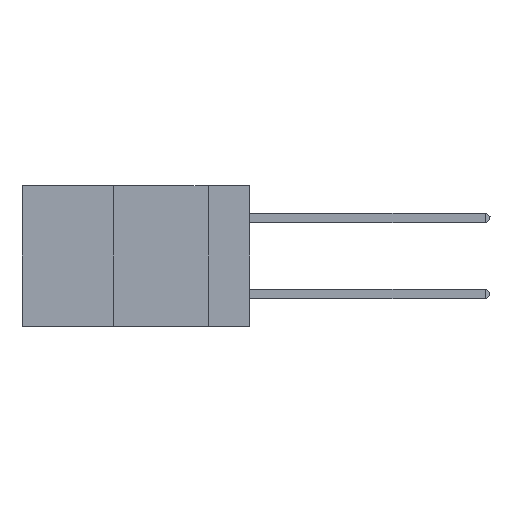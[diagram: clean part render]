
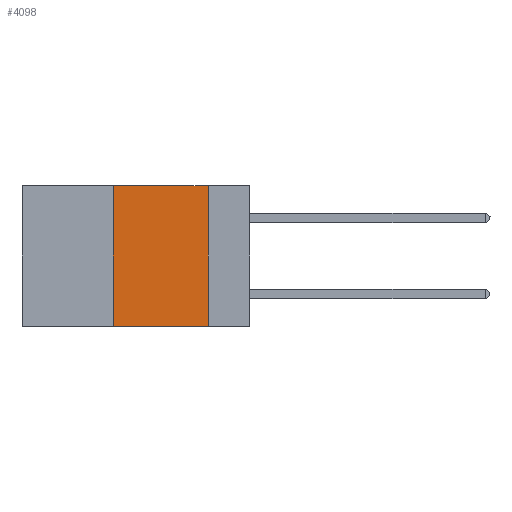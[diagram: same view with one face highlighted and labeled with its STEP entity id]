
A CAD part, left-side view. The second image highlights one B-rep face of the part: STEP entity #4098.
In plain terms, the highlighted planar face has unit normal (-1, 0, 0).
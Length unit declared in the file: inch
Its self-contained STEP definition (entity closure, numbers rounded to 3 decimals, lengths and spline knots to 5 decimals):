
#2350 = VERTEX_POINT ( 'NONE', #8051 ) ;
#2591 = EDGE_LOOP ( 'NONE', ( #5721, #17587, #22208, #9639 ) ) ;
#2905 = LINE ( 'NONE', #17346, #23417 ) ;
#4098 = ADVANCED_FACE ( 'NONE', ( #21473 ), #21972, .F. ) ;
#4658 = CARTESIAN_POINT ( 'NONE',  ( 0., 0.36, 0. ) ) ;
#5721 = ORIENTED_EDGE ( 'NONE', *, *, #7658, .F. ) ;
#7232 = DIRECTION ( 'NONE',  ( 0., -1., 0. ) ) ;
#7382 = EDGE_CURVE ( 'NONE', #23721, #17882, #17260, .T. ) ;
#7491 = CARTESIAN_POINT ( 'NONE',  ( 0., 0.6, 0. ) ) ;
#7658 = EDGE_CURVE ( 'NONE', #17882, #2350, #24293, .T. ) ;
#7689 = VECTOR ( 'NONE', #10602, 39.37008 ) ;
#8051 = CARTESIAN_POINT ( 'NONE',  ( 0., 0.11, -0.37 ) ) ;
#8154 = DIRECTION ( 'NONE',  ( 1., 0., 0. ) ) ;
#8380 = CARTESIAN_POINT ( 'NONE',  ( 0., 0.11, 0. ) ) ;
#9639 = ORIENTED_EDGE ( 'NONE', *, *, #20688, .T. ) ;
#9808 = AXIS2_PLACEMENT_3D ( 'NONE', #14433, #8154, #19993 ) ;
#10602 = DIRECTION ( 'NONE',  ( 0., 0., -1. ) ) ;
#12702 = CARTESIAN_POINT ( 'NONE',  ( 0., 0.36, -0.37 ) ) ;
#13387 = VERTEX_POINT ( 'NONE', #12702 ) ;
#13910 = VECTOR ( 'NONE', #15859, 39.37008 ) ;
#14433 = CARTESIAN_POINT ( 'NONE',  ( 0., 0.6, 0. ) ) ;
#15370 = EDGE_CURVE ( 'NONE', #13387, #23721, #2905, .T. ) ;
#15859 = DIRECTION ( 'NONE',  ( 0., -1., 0. ) ) ;
#17260 = LINE ( 'NONE', #7491, #18092 ) ;
#17346 = CARTESIAN_POINT ( 'NONE',  ( 0., 0.36, 0. ) ) ;
#17587 = ORIENTED_EDGE ( 'NONE', *, *, #7382, .F. ) ;
#17882 = VERTEX_POINT ( 'NONE', #25058 ) ;
#18092 = VECTOR ( 'NONE', #7232, 39.37008 ) ;
#19993 = DIRECTION ( 'NONE',  ( 0., 0., -1. ) ) ;
#20688 = EDGE_CURVE ( 'NONE', #13387, #2350, #22236, .T. ) ;
#21473 = FACE_OUTER_BOUND ( 'NONE', #2591, .T. ) ;
#21972 = PLANE ( 'NONE',  #9808 ) ;
#21979 = CARTESIAN_POINT ( 'NONE',  ( 0., 0.6, -0.37 ) ) ;
#22208 = ORIENTED_EDGE ( 'NONE', *, *, #15370, .F. ) ;
#22236 = LINE ( 'NONE', #21979, #13910 ) ;
#23417 = VECTOR ( 'NONE', #25691, 39.37008 ) ;
#23721 = VERTEX_POINT ( 'NONE', #4658 ) ;
#24293 = LINE ( 'NONE', #8380, #7689 ) ;
#25058 = CARTESIAN_POINT ( 'NONE',  ( 0., 0.11, 0. ) ) ;
#25691 = DIRECTION ( 'NONE',  ( 0., 0., 1. ) ) ;
